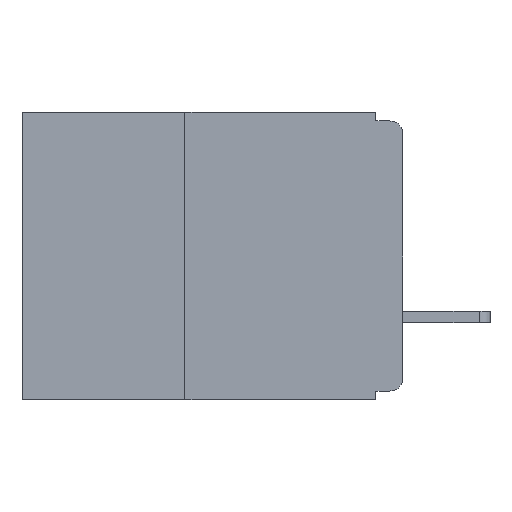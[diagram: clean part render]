
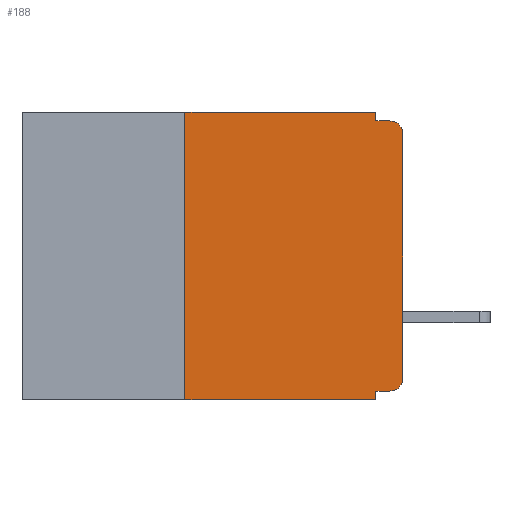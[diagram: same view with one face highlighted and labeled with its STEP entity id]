
A CAD part, left-side view. The second image highlights one B-rep face of the part: STEP entity #188.
In plain terms, the highlighted planar face has unit normal (-1, 0, 0).
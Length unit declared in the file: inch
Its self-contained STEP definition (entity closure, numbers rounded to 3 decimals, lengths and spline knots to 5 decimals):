
#151 = VERTEX_POINT ( 'NONE', #26675 ) ;
#188 = ADVANCED_FACE ( 'NONE', ( #29714 ), #26742, .F. ) ;
#476 = CARTESIAN_POINT ( 'NONE',  ( 0., 0.031, -0.01 ) ) ;
#501 = CARTESIAN_POINT ( 'NONE',  ( 0., 0.015, -0.305 ) ) ;
#543 = DIRECTION ( 'NONE',  ( 0., 0., 1. ) ) ;
#827 = VERTEX_POINT ( 'NONE', #21235 ) ;
#1590 = VECTOR ( 'NONE', #3101, 39.37008 ) ;
#1756 = VERTEX_POINT ( 'NONE', #8699 ) ;
#2710 = CARTESIAN_POINT ( 'NONE',  ( 0., 0., -0.305 ) ) ;
#2898 = DIRECTION ( 'NONE',  ( 0., 0., -1. ) ) ;
#3101 = DIRECTION ( 'NONE',  ( 0., 1., 0. ) ) ;
#4935 = EDGE_CURVE ( 'NONE', #8817, #28021, #25725, .T. ) ;
#4998 = AXIS2_PLACEMENT_3D ( 'NONE', #24419, #10797, #26754 ) ;
#5139 = CARTESIAN_POINT ( 'NONE',  ( 0., 0.031, -0.32 ) ) ;
#5183 = ORIENTED_EDGE ( 'NONE', *, *, #15262, .F. ) ;
#5710 = ORIENTED_EDGE ( 'NONE', *, *, #9635, .F. ) ;
#7285 = VECTOR ( 'NONE', #11868, 39.37008 ) ;
#7290 = CARTESIAN_POINT ( 'NONE',  ( 0., 0.437, 0. ) ) ;
#7520 = LINE ( 'NONE', #14484, #14328 ) ;
#7725 = CARTESIAN_POINT ( 'NONE',  ( 0., 0.25, 0. ) ) ;
#7726 = VECTOR ( 'NONE', #23218, 39.37008 ) ;
#7752 = EDGE_CURVE ( 'NONE', #1756, #827, #21280, .T. ) ;
#8699 = CARTESIAN_POINT ( 'NONE',  ( 0., 0., -0.025 ) ) ;
#8817 = VERTEX_POINT ( 'NONE', #9479 ) ;
#8919 = EDGE_CURVE ( 'NONE', #21637, #1756, #21077, .T. ) ;
#9479 = CARTESIAN_POINT ( 'NONE',  ( 0., 0.25, -0.33 ) ) ;
#9564 = CARTESIAN_POINT ( 'NONE',  ( 0., 0.437, -0.33 ) ) ;
#9635 = EDGE_CURVE ( 'NONE', #27210, #15156, #19248, .T. ) ;
#10219 = AXIS2_PLACEMENT_3D ( 'NONE', #501, #16694, #2898 ) ;
#10797 = DIRECTION ( 'NONE',  ( -1., 0., 0. ) ) ;
#11204 = LINE ( 'NONE', #15920, #15827 ) ;
#11868 = DIRECTION ( 'NONE',  ( 0., 0., 1. ) ) ;
#12385 = VECTOR ( 'NONE', #23843, 39.37008 ) ;
#12503 = CARTESIAN_POINT ( 'NONE',  ( 0., 0., -0.01 ) ) ;
#13031 = EDGE_CURVE ( 'NONE', #8817, #19873, #13391, .T. ) ;
#13391 = LINE ( 'NONE', #23176, #7285 ) ;
#13805 = LINE ( 'NONE', #14198, #7726 ) ;
#14198 = CARTESIAN_POINT ( 'NONE',  ( 0., 0.031, 0. ) ) ;
#14328 = VECTOR ( 'NONE', #18940, 39.37008 ) ;
#14484 = CARTESIAN_POINT ( 'NONE',  ( 0., 0.031, -0.33 ) ) ;
#15156 = VERTEX_POINT ( 'NONE', #5139 ) ;
#15262 = EDGE_CURVE ( 'NONE', #25094, #827, #24480, .T. ) ;
#15302 = AXIS2_PLACEMENT_3D ( 'NONE', #7290, #23153, #22767 ) ;
#15451 = ORIENTED_EDGE ( 'NONE', *, *, #27921, .T. ) ;
#15827 = VECTOR ( 'NONE', #18208, 39.37008 ) ;
#15920 = CARTESIAN_POINT ( 'NONE',  ( 0., 0.437, 0. ) ) ;
#16694 = DIRECTION ( 'NONE',  ( -1., 0., 0. ) ) ;
#16996 = CARTESIAN_POINT ( 'NONE',  ( 0., 0., -0.32 ) ) ;
#17490 = EDGE_CURVE ( 'NONE', #19873, #151, #11204, .T. ) ;
#18208 = DIRECTION ( 'NONE',  ( 0., -1., 0. ) ) ;
#18940 = DIRECTION ( 'NONE',  ( 0., 0., -1. ) ) ;
#19238 = ORIENTED_EDGE ( 'NONE', *, *, #17490, .F. ) ;
#19248 = LINE ( 'NONE', #16996, #1590 ) ;
#19251 = CARTESIAN_POINT ( 'NONE',  ( 0., 0.031, -0.33 ) ) ;
#19609 = ORIENTED_EDGE ( 'NONE', *, *, #13031, .F. ) ;
#19873 = VERTEX_POINT ( 'NONE', #7725 ) ;
#20287 = ORIENTED_EDGE ( 'NONE', *, *, #22111, .F. ) ;
#20348 = VECTOR ( 'NONE', #543, 39.37008 ) ;
#21061 = VECTOR ( 'NONE', #25488, 39.37008 ) ;
#21077 = LINE ( 'NONE', #28094, #20348 ) ;
#21235 = CARTESIAN_POINT ( 'NONE',  ( 0., 0.015, -0.01 ) ) ;
#21280 = CIRCLE ( 'NONE', #4998, 0.015 ) ;
#21637 = VERTEX_POINT ( 'NONE', #2710 ) ;
#22111 = EDGE_CURVE ( 'NONE', #151, #25094, #13805, .T. ) ;
#22767 = DIRECTION ( 'NONE',  ( 0., 0., -1. ) ) ;
#22864 = CIRCLE ( 'NONE', #10219, 0.015 ) ;
#23153 = DIRECTION ( 'NONE',  ( 1., 0., 0. ) ) ;
#23176 = CARTESIAN_POINT ( 'NONE',  ( 0., 0.25, -0.33 ) ) ;
#23218 = DIRECTION ( 'NONE',  ( 0., 0., -1. ) ) ;
#23843 = DIRECTION ( 'NONE',  ( 0., -1., 0. ) ) ;
#24419 = CARTESIAN_POINT ( 'NONE',  ( 0., 0.015, -0.025 ) ) ;
#24480 = LINE ( 'NONE', #12503, #12385 ) ;
#25094 = VERTEX_POINT ( 'NONE', #476 ) ;
#25126 = EDGE_CURVE ( 'NONE', #15156, #28021, #7520, .T. ) ;
#25488 = DIRECTION ( 'NONE',  ( 0., -1., 0. ) ) ;
#25595 = ORIENTED_EDGE ( 'NONE', *, *, #8919, .T. ) ;
#25725 = LINE ( 'NONE', #9564, #21061 ) ;
#26115 = ORIENTED_EDGE ( 'NONE', *, *, #25126, .F. ) ;
#26255 = EDGE_LOOP ( 'NONE', ( #25595, #28444, #5183, #20287, #19238, #19609, #28605, #26115, #5710, #15451 ) ) ;
#26675 = CARTESIAN_POINT ( 'NONE',  ( 0., 0.031, 0. ) ) ;
#26742 = PLANE ( 'NONE',  #15302 ) ;
#26754 = DIRECTION ( 'NONE',  ( 0., 0., -1. ) ) ;
#27210 = VERTEX_POINT ( 'NONE', #29365 ) ;
#27921 = EDGE_CURVE ( 'NONE', #27210, #21637, #22864, .T. ) ;
#28021 = VERTEX_POINT ( 'NONE', #19251 ) ;
#28094 = CARTESIAN_POINT ( 'NONE',  ( 0., 0., 0. ) ) ;
#28444 = ORIENTED_EDGE ( 'NONE', *, *, #7752, .T. ) ;
#28605 = ORIENTED_EDGE ( 'NONE', *, *, #4935, .T. ) ;
#29365 = CARTESIAN_POINT ( 'NONE',  ( 0., 0.015, -0.32 ) ) ;
#29714 = FACE_OUTER_BOUND ( 'NONE', #26255, .T. ) ;
